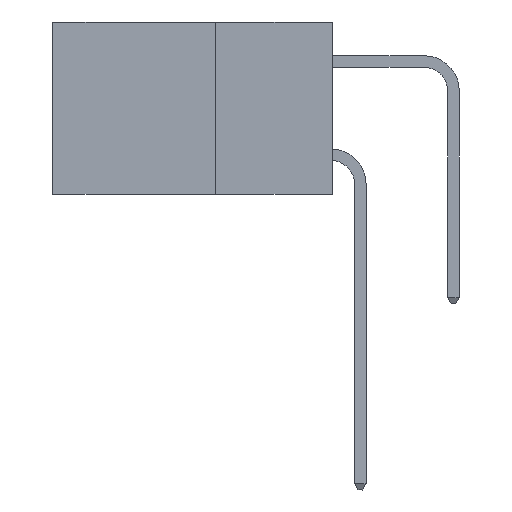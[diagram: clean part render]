
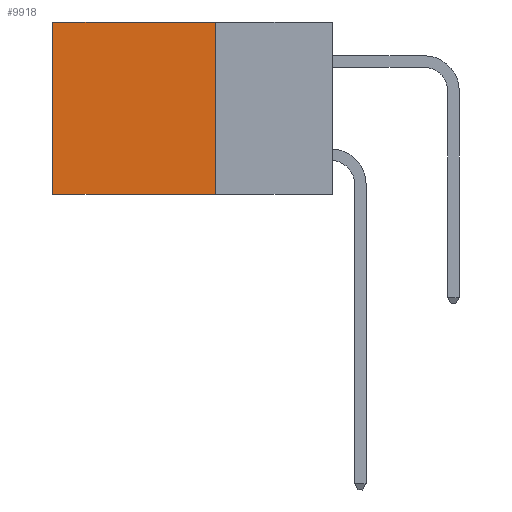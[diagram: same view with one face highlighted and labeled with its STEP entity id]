
A CAD part, left-side view. The second image highlights one B-rep face of the part: STEP entity #9918.
In plain terms, the highlighted planar face has unit normal (-1, 0, 0).
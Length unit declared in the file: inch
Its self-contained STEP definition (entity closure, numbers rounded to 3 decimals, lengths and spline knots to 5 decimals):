
#568 = DIRECTION ( 'NONE',  ( 0., 0., -1. ) ) ;
#946 = ORIENTED_EDGE ( 'NONE', *, *, #4387, .T. ) ;
#1199 = ORIENTED_EDGE ( 'NONE', *, *, #12253, .F. ) ;
#1329 = DIRECTION ( 'NONE',  ( 0., 0., -1. ) ) ;
#1622 = ORIENTED_EDGE ( 'NONE', *, *, #3506, .T. ) ;
#1638 = ORIENTED_EDGE ( 'NONE', *, *, #11086, .F. ) ;
#2307 = CARTESIAN_POINT ( 'NONE',  ( 0.298, 0.25, -0.37 ) ) ;
#3257 = LINE ( 'NONE', #2307, #5668 ) ;
#3455 = VECTOR ( 'NONE', #5774, 39.37008 ) ;
#3506 = EDGE_CURVE ( 'NONE', #5005, #9115, #8900, .T. ) ;
#4317 = CARTESIAN_POINT ( 'NONE',  ( 0.298, 0.25, 0. ) ) ;
#4375 = CARTESIAN_POINT ( 'NONE',  ( 0.298, 0.25, 0. ) ) ;
#4387 = EDGE_CURVE ( 'NONE', #9115, #6828, #11391, .T. ) ;
#4987 = CARTESIAN_POINT ( 'NONE',  ( 0.298, 0.6, -0.37 ) ) ;
#5005 = VERTEX_POINT ( 'NONE', #4317 ) ;
#5145 = DIRECTION ( 'NONE',  ( 0., 0., -1. ) ) ;
#5166 = FACE_OUTER_BOUND ( 'NONE', #10237, .T. ) ;
#5668 = VECTOR ( 'NONE', #7472, 39.37008 ) ;
#5774 = DIRECTION ( 'NONE',  ( 0., 1., 0. ) ) ;
#6828 = VERTEX_POINT ( 'NONE', #4987 ) ;
#7472 = DIRECTION ( 'NONE',  ( 0., 1., 0. ) ) ;
#7559 = DIRECTION ( 'NONE',  ( 1., 0., 0. ) ) ;
#7853 = VERTEX_POINT ( 'NONE', #10525 ) ;
#8466 = AXIS2_PLACEMENT_3D ( 'NONE', #9548, #7559, #1329 ) ;
#8900 = LINE ( 'NONE', #4375, #3455 ) ;
#9115 = VERTEX_POINT ( 'NONE', #11805 ) ;
#9241 = VECTOR ( 'NONE', #568, 39.37008 ) ;
#9548 = CARTESIAN_POINT ( 'NONE',  ( 0.298, 0.25, 0. ) ) ;
#9918 = ADVANCED_FACE ( 'NONE', ( #5166 ), #11549, .F. ) ;
#10078 = LINE ( 'NONE', #12677, #9241 ) ;
#10237 = EDGE_LOOP ( 'NONE', ( #946, #1199, #1638, #1622 ) ) ;
#10525 = CARTESIAN_POINT ( 'NONE',  ( 0.298, 0.25, -0.37 ) ) ;
#10797 = VECTOR ( 'NONE', #5145, 39.37008 ) ;
#11086 = EDGE_CURVE ( 'NONE', #5005, #7853, #10078, .T. ) ;
#11391 = LINE ( 'NONE', #12996, #10797 ) ;
#11549 = PLANE ( 'NONE',  #8466 ) ;
#11805 = CARTESIAN_POINT ( 'NONE',  ( 0.298, 0.6, 0. ) ) ;
#12253 = EDGE_CURVE ( 'NONE', #7853, #6828, #3257, .T. ) ;
#12677 = CARTESIAN_POINT ( 'NONE',  ( 0.298, 0.25, 0. ) ) ;
#12996 = CARTESIAN_POINT ( 'NONE',  ( 0.298, 0.6, 0. ) ) ;
